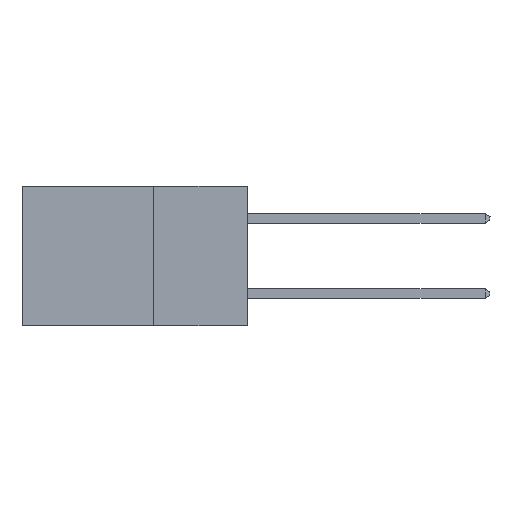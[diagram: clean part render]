
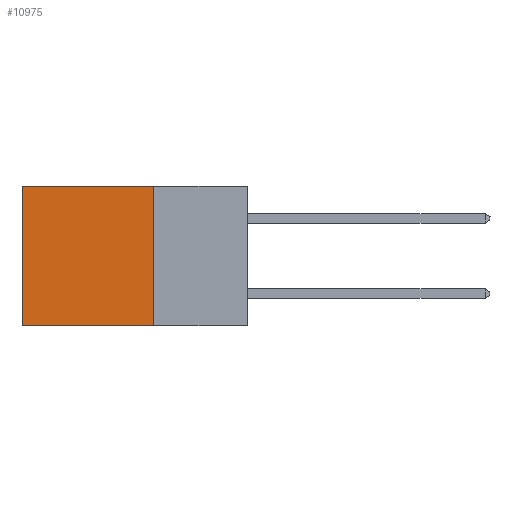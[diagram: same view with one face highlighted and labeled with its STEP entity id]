
A CAD part, left-side view. The second image highlights one B-rep face of the part: STEP entity #10975.
In plain terms, the highlighted planar face has unit normal (-1, 0, 0).
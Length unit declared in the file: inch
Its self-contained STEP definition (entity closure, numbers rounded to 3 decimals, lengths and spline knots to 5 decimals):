
#178 = LINE ( 'NONE', #10406, #810 ) ;
#237 = DIRECTION ( 'NONE',  ( 0., 1., 0. ) ) ;
#516 = CARTESIAN_POINT ( 'NONE',  ( 0.2615, 0.25, 0. ) ) ;
#790 = CARTESIAN_POINT ( 'NONE',  ( 0.2615, 0.25, -0.37 ) ) ;
#810 = VECTOR ( 'NONE', #2122, 39.37008 ) ;
#889 = DIRECTION ( 'NONE',  ( 0., 0., -1. ) ) ;
#1151 = ORIENTED_EDGE ( 'NONE', *, *, #2210, .F. ) ;
#1561 = EDGE_CURVE ( 'NONE', #10883, #10136, #2807, .T. ) ;
#1710 = PLANE ( 'NONE',  #5532 ) ;
#2034 = DIRECTION ( 'NONE',  ( 0., 0., -1. ) ) ;
#2067 = VECTOR ( 'NONE', #2034, 39.37008 ) ;
#2122 = DIRECTION ( 'NONE',  ( 0., 1., 0. ) ) ;
#2210 = EDGE_CURVE ( 'NONE', #10136, #7859, #178, .T. ) ;
#2257 = LINE ( 'NONE', #13431, #2067 ) ;
#2340 = CARTESIAN_POINT ( 'NONE',  ( 0.2615, 0.25, 0. ) ) ;
#2807 = LINE ( 'NONE', #10591, #7221 ) ;
#2972 = VERTEX_POINT ( 'NONE', #4469 ) ;
#3949 = DIRECTION ( 'NONE',  ( 0., 0., -1. ) ) ;
#4469 = CARTESIAN_POINT ( 'NONE',  ( 0.2615, 0.6, 0. ) ) ;
#4619 = CARTESIAN_POINT ( 'NONE',  ( 0.2615, 0.6, -0.37 ) ) ;
#5392 = EDGE_CURVE ( 'NONE', #2972, #7859, #2257, .T. ) ;
#5532 = AXIS2_PLACEMENT_3D ( 'NONE', #11019, #14373, #889 ) ;
#6574 = FACE_OUTER_BOUND ( 'NONE', #13229, .T. ) ;
#7221 = VECTOR ( 'NONE', #3949, 39.37008 ) ;
#7676 = VECTOR ( 'NONE', #237, 39.37008 ) ;
#7859 = VERTEX_POINT ( 'NONE', #4619 ) ;
#8346 = ORIENTED_EDGE ( 'NONE', *, *, #1561, .F. ) ;
#10136 = VERTEX_POINT ( 'NONE', #790 ) ;
#10406 = CARTESIAN_POINT ( 'NONE',  ( 0.2615, 0.25, -0.37 ) ) ;
#10591 = CARTESIAN_POINT ( 'NONE',  ( 0.2615, 0.25, -0.37 ) ) ;
#10883 = VERTEX_POINT ( 'NONE', #516 ) ;
#10975 = ADVANCED_FACE ( 'NONE', ( #6574 ), #1710, .F. ) ;
#11019 = CARTESIAN_POINT ( 'NONE',  ( 0.2615, 0.25, -0.37 ) ) ;
#11636 = ORIENTED_EDGE ( 'NONE', *, *, #5392, .T. ) ;
#12179 = EDGE_CURVE ( 'NONE', #10883, #2972, #12564, .T. ) ;
#12564 = LINE ( 'NONE', #2340, #7676 ) ;
#13229 = EDGE_LOOP ( 'NONE', ( #11636, #1151, #8346, #14594 ) ) ;
#13431 = CARTESIAN_POINT ( 'NONE',  ( 0.2615, 0.6, -0.37 ) ) ;
#14373 = DIRECTION ( 'NONE',  ( 1., 0., 0. ) ) ;
#14594 = ORIENTED_EDGE ( 'NONE', *, *, #12179, .T. ) ;
